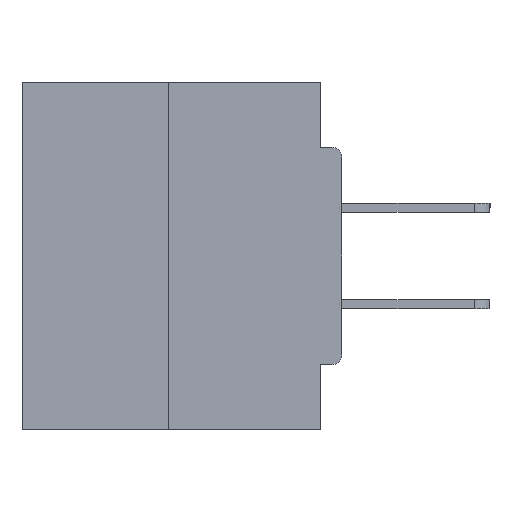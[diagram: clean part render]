
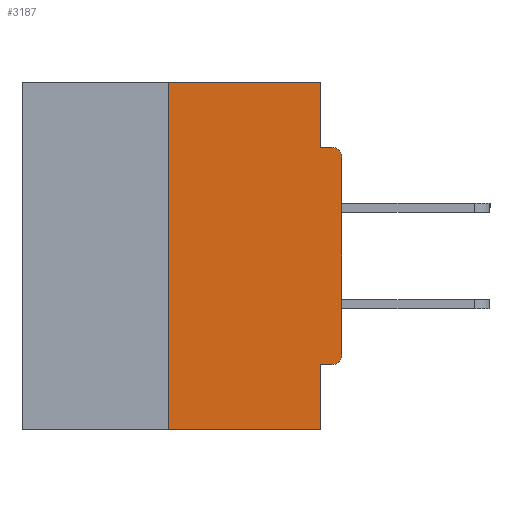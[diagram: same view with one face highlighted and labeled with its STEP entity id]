
A CAD part, left-side view. The second image highlights one B-rep face of the part: STEP entity #3187.
In plain terms, the highlighted planar face has unit normal (-1, 0, 0).
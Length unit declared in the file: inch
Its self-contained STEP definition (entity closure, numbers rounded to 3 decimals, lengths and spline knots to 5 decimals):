
#1 = CARTESIAN_POINT ( 'NONE',  ( 0., 0., -0.0935 ) ) ;
#166 = CARTESIAN_POINT ( 'NONE',  ( 0., 0.031, 0. ) ) ;
#1273 = EDGE_CURVE ( 'NONE', #1282, #16136, #24383, .T. ) ;
#1282 = VERTEX_POINT ( 'NONE', #15549 ) ;
#1522 = VECTOR ( 'NONE', #21977, 39.37008 ) ;
#2273 = CARTESIAN_POINT ( 'NONE',  ( 0., 0.031, -0.4065 ) ) ;
#2420 = LINE ( 'NONE', #13447, #33465 ) ;
#2862 = CARTESIAN_POINT ( 'NONE',  ( 0., 0.015, -0.0935 ) ) ;
#3036 = CARTESIAN_POINT ( 'NONE',  ( 0., 0.46, 0. ) ) ;
#3187 = ADVANCED_FACE ( 'NONE', ( #3371 ), #20603, .F. ) ;
#3371 = FACE_OUTER_BOUND ( 'NONE', #9112, .T. ) ;
#3824 = VECTOR ( 'NONE', #30737, 39.37008 ) ;
#5152 = CIRCLE ( 'NONE', #21587, 0.015 ) ;
#5764 = VERTEX_POINT ( 'NONE', #11629 ) ;
#5867 = ORIENTED_EDGE ( 'NONE', *, *, #32459, .F. ) ;
#6341 = CARTESIAN_POINT ( 'NONE',  ( 0., 0.031, -0.5 ) ) ;
#6461 = ORIENTED_EDGE ( 'NONE', *, *, #29164, .F. ) ;
#6619 = CARTESIAN_POINT ( 'NONE',  ( 0., 0.015, -0.1085 ) ) ;
#7132 = DIRECTION ( 'NONE',  ( 0., 0., -1. ) ) ;
#7187 = AXIS2_PLACEMENT_3D ( 'NONE', #17917, #30831, #7132 ) ;
#7249 = EDGE_CURVE ( 'NONE', #16136, #9066, #29903, .T. ) ;
#7570 = CARTESIAN_POINT ( 'NONE',  ( 0., 0., 0. ) ) ;
#8826 = VERTEX_POINT ( 'NONE', #2273 ) ;
#9066 = VERTEX_POINT ( 'NONE', #2862 ) ;
#9112 = EDGE_LOOP ( 'NONE', ( #6461, #17330, #12288, #21065, #5867, #28486, #11893, #21128, #11631, #20456 ) ) ;
#9533 = VECTOR ( 'NONE', #13302, 39.37008 ) ;
#10140 = CARTESIAN_POINT ( 'NONE',  ( 0., 0.25, 0. ) ) ;
#10804 = CARTESIAN_POINT ( 'NONE',  ( 0., 0., -0.1085 ) ) ;
#11293 = DIRECTION ( 'NONE',  ( 0., 1., 0. ) ) ;
#11375 = LINE ( 'NONE', #22152, #3824 ) ;
#11629 = CARTESIAN_POINT ( 'NONE',  ( 0., 0.25, -0.5 ) ) ;
#11631 = ORIENTED_EDGE ( 'NONE', *, *, #25544, .F. ) ;
#11893 = ORIENTED_EDGE ( 'NONE', *, *, #1273, .T. ) ;
#12068 = DIRECTION ( 'NONE',  ( 0., -1., 0. ) ) ;
#12111 = LINE ( 'NONE', #24505, #12510 ) ;
#12182 = CARTESIAN_POINT ( 'NONE',  ( 0., 0.46, -0.5 ) ) ;
#12288 = ORIENTED_EDGE ( 'NONE', *, *, #22372, .T. ) ;
#12510 = VECTOR ( 'NONE', #11293, 39.37008 ) ;
#13302 = DIRECTION ( 'NONE',  ( 0., 0., 1. ) ) ;
#13447 = CARTESIAN_POINT ( 'NONE',  ( 0., 0.031, 0. ) ) ;
#13878 = VECTOR ( 'NONE', #18920, 39.37008 ) ;
#15549 = CARTESIAN_POINT ( 'NONE',  ( 0., 0., -0.3915 ) ) ;
#15577 = LINE ( 'NONE', #1, #13878 ) ;
#16136 = VERTEX_POINT ( 'NONE', #10804 ) ;
#16574 = EDGE_CURVE ( 'NONE', #29248, #29111, #2420, .T. ) ;
#17301 = VERTEX_POINT ( 'NONE', #25537 ) ;
#17330 = ORIENTED_EDGE ( 'NONE', *, *, #33224, .F. ) ;
#17917 = CARTESIAN_POINT ( 'NONE',  ( 0., 0.46, 0. ) ) ;
#18920 = DIRECTION ( 'NONE',  ( 0., -1., 0. ) ) ;
#19069 = VERTEX_POINT ( 'NONE', #10140 ) ;
#20456 = ORIENTED_EDGE ( 'NONE', *, *, #16574, .F. ) ;
#20475 = VECTOR ( 'NONE', #12068, 39.37008 ) ;
#20603 = PLANE ( 'NONE',  #7187 ) ;
#21065 = ORIENTED_EDGE ( 'NONE', *, *, #25785, .F. ) ;
#21128 = ORIENTED_EDGE ( 'NONE', *, *, #7249, .T. ) ;
#21540 = VERTEX_POINT ( 'NONE', #6341 ) ;
#21587 = AXIS2_PLACEMENT_3D ( 'NONE', #30305, #24989, #27463 ) ;
#21771 = DIRECTION ( 'NONE',  ( 0., 0., -1. ) ) ;
#21977 = DIRECTION ( 'NONE',  ( 0., -1., 0. ) ) ;
#22152 = CARTESIAN_POINT ( 'NONE',  ( 0., 0.031, -0.5 ) ) ;
#22372 = EDGE_CURVE ( 'NONE', #5764, #21540, #25506, .T. ) ;
#24383 = LINE ( 'NONE', #7570, #29499 ) ;
#24505 = CARTESIAN_POINT ( 'NONE',  ( 0., 0., -0.4065 ) ) ;
#24980 = LINE ( 'NONE', #3036, #1522 ) ;
#24989 = DIRECTION ( 'NONE',  ( -1., 0., 0. ) ) ;
#25114 = EDGE_CURVE ( 'NONE', #17301, #1282, #5152, .T. ) ;
#25506 = LINE ( 'NONE', #12182, #20475 ) ;
#25537 = CARTESIAN_POINT ( 'NONE',  ( 0., 0.015, -0.4065 ) ) ;
#25544 = EDGE_CURVE ( 'NONE', #29111, #9066, #15577, .T. ) ;
#25785 = EDGE_CURVE ( 'NONE', #8826, #21540, #11375, .T. ) ;
#27463 = DIRECTION ( 'NONE',  ( 0., 0., -1. ) ) ;
#27942 = DIRECTION ( 'NONE',  ( 0., 0., -1. ) ) ;
#28486 = ORIENTED_EDGE ( 'NONE', *, *, #25114, .T. ) ;
#29111 = VERTEX_POINT ( 'NONE', #32795 ) ;
#29164 = EDGE_CURVE ( 'NONE', #19069, #29248, #24980, .T. ) ;
#29248 = VERTEX_POINT ( 'NONE', #166 ) ;
#29499 = VECTOR ( 'NONE', #34452, 39.37008 ) ;
#29755 = CARTESIAN_POINT ( 'NONE',  ( 0., 0.25, 0. ) ) ;
#29903 = CIRCLE ( 'NONE', #33339, 0.015 ) ;
#30305 = CARTESIAN_POINT ( 'NONE',  ( 0., 0.015, -0.3915 ) ) ;
#30496 = LINE ( 'NONE', #29755, #9533 ) ;
#30737 = DIRECTION ( 'NONE',  ( 0., 0., -1. ) ) ;
#30831 = DIRECTION ( 'NONE',  ( 1., 0., 0. ) ) ;
#32459 = EDGE_CURVE ( 'NONE', #17301, #8826, #12111, .T. ) ;
#32795 = CARTESIAN_POINT ( 'NONE',  ( 0., 0.031, -0.0935 ) ) ;
#33127 = DIRECTION ( 'NONE',  ( -1., 0., 0. ) ) ;
#33224 = EDGE_CURVE ( 'NONE', #5764, #19069, #30496, .T. ) ;
#33339 = AXIS2_PLACEMENT_3D ( 'NONE', #6619, #33127, #27942 ) ;
#33465 = VECTOR ( 'NONE', #21771, 39.37008 ) ;
#34452 = DIRECTION ( 'NONE',  ( 0., 0., 1. ) ) ;
